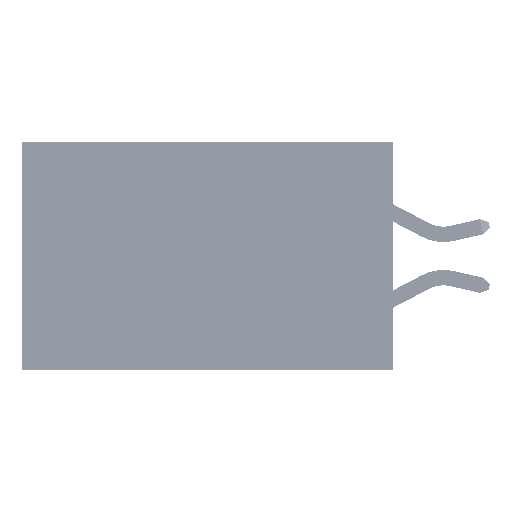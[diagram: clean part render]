
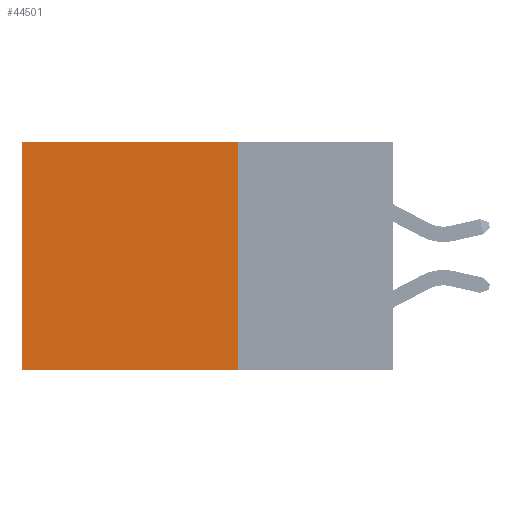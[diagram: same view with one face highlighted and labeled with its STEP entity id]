
A CAD part, left-side view. The second image highlights one B-rep face of the part: STEP entity #44501.
In plain terms, the highlighted planar face has unit normal (-1, 0, 0).
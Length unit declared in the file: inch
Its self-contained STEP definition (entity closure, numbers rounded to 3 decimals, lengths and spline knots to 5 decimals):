
#272 = LINE ( 'NONE', #25654, #38090 ) ;
#1469 = EDGE_CURVE ( 'NONE', #6879, #6067, #2020, .T. ) ;
#2020 = LINE ( 'NONE', #43708, #5447 ) ;
#3006 = VECTOR ( 'NONE', #8690, 39.37008 ) ;
#4104 = AXIS2_PLACEMENT_3D ( 'NONE', #19354, #26733, #15843 ) ;
#5447 = VECTOR ( 'NONE', #29016, 39.37008 ) ;
#6067 = VERTEX_POINT ( 'NONE', #33526 ) ;
#6879 = VERTEX_POINT ( 'NONE', #16912 ) ;
#8690 = DIRECTION ( 'NONE',  ( 0., 0., -1. ) ) ;
#13691 = EDGE_CURVE ( 'NONE', #30351, #20182, #17305, .T. ) ;
#15022 = EDGE_LOOP ( 'NONE', ( #32040, #42218, #32638, #36347 ) ) ;
#15843 = DIRECTION ( 'NONE',  ( 0., 0., -1. ) ) ;
#16453 = FACE_OUTER_BOUND ( 'NONE', #15022, .T. ) ;
#16766 = LINE ( 'NONE', #19593, #3006 ) ;
#16912 = CARTESIAN_POINT ( 'NONE',  ( 0.2875, 0.25, 0. ) ) ;
#17305 = LINE ( 'NONE', #39601, #43047 ) ;
#19354 = CARTESIAN_POINT ( 'NONE',  ( 0.2875, 0.25, 0. ) ) ;
#19593 = CARTESIAN_POINT ( 'NONE',  ( 0.2875, 0.25, 0. ) ) ;
#20182 = VERTEX_POINT ( 'NONE', #42909 ) ;
#20777 = EDGE_CURVE ( 'NONE', #6879, #30351, #16766, .T. ) ;
#22409 = DIRECTION ( 'NONE',  ( 0., 1., 0. ) ) ;
#25335 = CARTESIAN_POINT ( 'NONE',  ( 0.2875, 0.25, -0.37 ) ) ;
#25654 = CARTESIAN_POINT ( 'NONE',  ( 0.2875, 0.6, 0. ) ) ;
#26733 = DIRECTION ( 'NONE',  ( 1., 0., 0. ) ) ;
#29016 = DIRECTION ( 'NONE',  ( 0., 1., 0. ) ) ;
#30351 = VERTEX_POINT ( 'NONE', #25335 ) ;
#32040 = ORIENTED_EDGE ( 'NONE', *, *, #40884, .T. ) ;
#32638 = ORIENTED_EDGE ( 'NONE', *, *, #20777, .F. ) ;
#33526 = CARTESIAN_POINT ( 'NONE',  ( 0.2875, 0.6, 0. ) ) ;
#36347 = ORIENTED_EDGE ( 'NONE', *, *, #1469, .T. ) ;
#38090 = VECTOR ( 'NONE', #40367, 39.37008 ) ;
#39601 = CARTESIAN_POINT ( 'NONE',  ( 0.2875, 0.25, -0.37 ) ) ;
#40367 = DIRECTION ( 'NONE',  ( 0., 0., -1. ) ) ;
#40884 = EDGE_CURVE ( 'NONE', #6067, #20182, #272, .T. ) ;
#42218 = ORIENTED_EDGE ( 'NONE', *, *, #13691, .F. ) ;
#42909 = CARTESIAN_POINT ( 'NONE',  ( 0.2875, 0.6, -0.37 ) ) ;
#43047 = VECTOR ( 'NONE', #22409, 39.37008 ) ;
#43708 = CARTESIAN_POINT ( 'NONE',  ( 0.2875, 0.25, 0. ) ) ;
#44501 = ADVANCED_FACE ( 'NONE', ( #16453 ), #45117, .F. ) ;
#45117 = PLANE ( 'NONE',  #4104 ) ;
